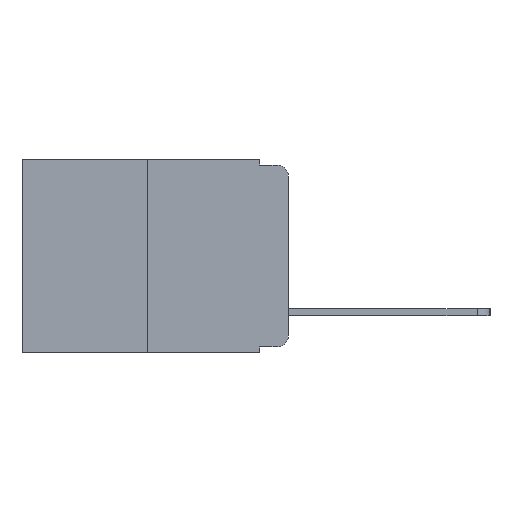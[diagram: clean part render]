
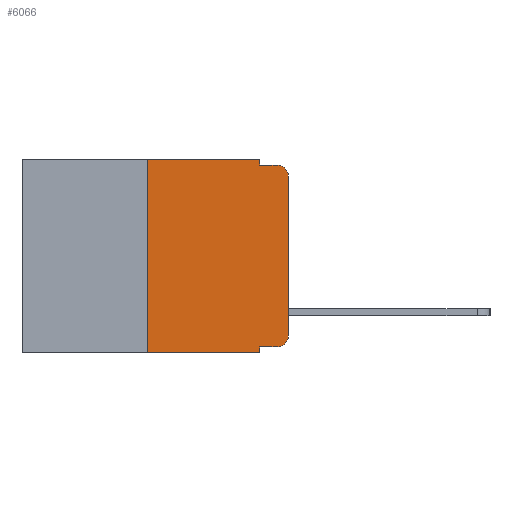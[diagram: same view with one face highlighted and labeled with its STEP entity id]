
A CAD part, left-side view. The second image highlights one B-rep face of the part: STEP entity #6066.
In plain terms, the highlighted planar face has unit normal (-1, 0, 0).
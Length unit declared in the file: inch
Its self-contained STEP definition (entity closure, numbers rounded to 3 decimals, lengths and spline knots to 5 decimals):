
#48 = DIRECTION ( 'NONE',  ( 0., 0., -1. ) ) ;
#591 = CARTESIAN_POINT ( 'NONE',  ( 0., 0.25, 0. ) ) ;
#1224 = FACE_OUTER_BOUND ( 'NONE', #18840, .T. ) ;
#1484 = DIRECTION ( 'NONE',  ( -1., 0., 0. ) ) ;
#1769 = CARTESIAN_POINT ( 'NONE',  ( 0., 0.051, -0.343 ) ) ;
#2409 = CARTESIAN_POINT ( 'NONE',  ( 0., 0.051, -0.01 ) ) ;
#2458 = EDGE_CURVE ( 'NONE', #11370, #16845, #17427, .T. ) ;
#2472 = ORIENTED_EDGE ( 'NONE', *, *, #4393, .F. ) ;
#2564 = CARTESIAN_POINT ( 'NONE',  ( 0., 0.051, -0.333 ) ) ;
#2819 = EDGE_CURVE ( 'NONE', #16101, #14282, #22959, .T. ) ;
#3037 = CARTESIAN_POINT ( 'NONE',  ( 0., 0.25, 0. ) ) ;
#3091 = CARTESIAN_POINT ( 'NONE',  ( 0., 0.02, -0.03 ) ) ;
#3475 = CIRCLE ( 'NONE', #16559, 0.02 ) ;
#3492 = CARTESIAN_POINT ( 'NONE',  ( 0., 0.02, -0.313 ) ) ;
#3577 = VECTOR ( 'NONE', #8615, 39.37008 ) ;
#3598 = ORIENTED_EDGE ( 'NONE', *, *, #7155, .F. ) ;
#4329 = ORIENTED_EDGE ( 'NONE', *, *, #2819, .F. ) ;
#4393 = EDGE_CURVE ( 'NONE', #19712, #17737, #8605, .T. ) ;
#4624 = CARTESIAN_POINT ( 'NONE',  ( 0., 0.02, -0.333 ) ) ;
#4773 = LINE ( 'NONE', #22912, #3577 ) ;
#4938 = DIRECTION ( 'NONE',  ( 0., 0., -1. ) ) ;
#5077 = ORIENTED_EDGE ( 'NONE', *, *, #21540, .T. ) ;
#5324 = EDGE_CURVE ( 'NONE', #16101, #6814, #19083, .T. ) ;
#5384 = CARTESIAN_POINT ( 'NONE',  ( 0., 0.02, -0.01 ) ) ;
#5534 = DIRECTION ( 'NONE',  ( 0., 0., -1. ) ) ;
#5817 = VECTOR ( 'NONE', #5534, 39.37008 ) ;
#6066 = ADVANCED_FACE ( 'NONE', ( #1224 ), #9665, .F. ) ;
#6263 = EDGE_CURVE ( 'NONE', #10305, #11370, #4773, .T. ) ;
#6814 = VERTEX_POINT ( 'NONE', #1769 ) ;
#7065 = ORIENTED_EDGE ( 'NONE', *, *, #15087, .F. ) ;
#7155 = EDGE_CURVE ( 'NONE', #8163, #19712, #21661, .T. ) ;
#7375 = VECTOR ( 'NONE', #8160, 39.37008 ) ;
#7403 = LINE ( 'NONE', #23131, #12507 ) ;
#8070 = VECTOR ( 'NONE', #18226, 39.37008 ) ;
#8160 = DIRECTION ( 'NONE',  ( 0., -1., 0. ) ) ;
#8163 = VERTEX_POINT ( 'NONE', #21022 ) ;
#8605 = LINE ( 'NONE', #2409, #7375 ) ;
#8615 = DIRECTION ( 'NONE',  ( 0., -1., 0. ) ) ;
#8666 = VECTOR ( 'NONE', #18124, 39.37008 ) ;
#9665 = PLANE ( 'NONE',  #14597 ) ;
#9990 = CARTESIAN_POINT ( 'NONE',  ( 0., 0., -0.313 ) ) ;
#10305 = VERTEX_POINT ( 'NONE', #2564 ) ;
#10750 = ORIENTED_EDGE ( 'NONE', *, *, #5324, .T. ) ;
#10871 = DIRECTION ( 'NONE',  ( 0., -1., 0. ) ) ;
#11062 = LINE ( 'NONE', #16855, #5817 ) ;
#11370 = VERTEX_POINT ( 'NONE', #4624 ) ;
#11606 = DIRECTION ( 'NONE',  ( 1., 0., 0. ) ) ;
#11610 = DIRECTION ( 'NONE',  ( 0., 0., -1. ) ) ;
#11843 = DIRECTION ( 'NONE',  ( 0., -1., 0. ) ) ;
#11847 = CARTESIAN_POINT ( 'NONE',  ( 0., 0.25, -0.343 ) ) ;
#12354 = VECTOR ( 'NONE', #23266, 39.37008 ) ;
#12507 = VECTOR ( 'NONE', #10871, 39.37008 ) ;
#12655 = AXIS2_PLACEMENT_3D ( 'NONE', #3492, #1484, #11610 ) ;
#13545 = CARTESIAN_POINT ( 'NONE',  ( 0., 0.051, -0.01 ) ) ;
#14282 = VERTEX_POINT ( 'NONE', #3037 ) ;
#14460 = VECTOR ( 'NONE', #11843, 39.37008 ) ;
#14597 = AXIS2_PLACEMENT_3D ( 'NONE', #22091, #11606, #48 ) ;
#14808 = ORIENTED_EDGE ( 'NONE', *, *, #15961, .F. ) ;
#15056 = EDGE_CURVE ( 'NONE', #16876, #17737, #3475, .T. ) ;
#15087 = EDGE_CURVE ( 'NONE', #14282, #8163, #7403, .T. ) ;
#15648 = CARTESIAN_POINT ( 'NONE',  ( 0., 0., -0.03 ) ) ;
#15794 = ORIENTED_EDGE ( 'NONE', *, *, #15056, .T. ) ;
#15961 = EDGE_CURVE ( 'NONE', #10305, #6814, #11062, .T. ) ;
#16101 = VERTEX_POINT ( 'NONE', #11847 ) ;
#16307 = DIRECTION ( 'NONE',  ( -1., 0., 0. ) ) ;
#16512 = CARTESIAN_POINT ( 'NONE',  ( 0., 0.051, 0. ) ) ;
#16559 = AXIS2_PLACEMENT_3D ( 'NONE', #3091, #16307, #4938 ) ;
#16845 = VERTEX_POINT ( 'NONE', #9990 ) ;
#16855 = CARTESIAN_POINT ( 'NONE',  ( 0., 0.051, 0. ) ) ;
#16876 = VERTEX_POINT ( 'NONE', #15648 ) ;
#17427 = CIRCLE ( 'NONE', #12655, 0.02 ) ;
#17737 = VERTEX_POINT ( 'NONE', #5384 ) ;
#18113 = ORIENTED_EDGE ( 'NONE', *, *, #6263, .T. ) ;
#18124 = DIRECTION ( 'NONE',  ( 0., 0., 1. ) ) ;
#18226 = DIRECTION ( 'NONE',  ( 0., 0., 1. ) ) ;
#18840 = EDGE_LOOP ( 'NONE', ( #5077, #15794, #2472, #3598, #7065, #4329, #10750, #14808, #18113, #23127 ) ) ;
#19083 = LINE ( 'NONE', #22314, #14460 ) ;
#19712 = VERTEX_POINT ( 'NONE', #13545 ) ;
#21022 = CARTESIAN_POINT ( 'NONE',  ( 0., 0.051, 0. ) ) ;
#21540 = EDGE_CURVE ( 'NONE', #16845, #16876, #21837, .T. ) ;
#21661 = LINE ( 'NONE', #16512, #12354 ) ;
#21837 = LINE ( 'NONE', #23133, #8666 ) ;
#22091 = CARTESIAN_POINT ( 'NONE',  ( 0., 0.473, 0. ) ) ;
#22314 = CARTESIAN_POINT ( 'NONE',  ( 0., 0.473, -0.343 ) ) ;
#22912 = CARTESIAN_POINT ( 'NONE',  ( 0., 0.051, -0.333 ) ) ;
#22959 = LINE ( 'NONE', #591, #8070 ) ;
#23127 = ORIENTED_EDGE ( 'NONE', *, *, #2458, .T. ) ;
#23131 = CARTESIAN_POINT ( 'NONE',  ( 0., 0.473, 0. ) ) ;
#23133 = CARTESIAN_POINT ( 'NONE',  ( 0., 0., 0. ) ) ;
#23266 = DIRECTION ( 'NONE',  ( 0., 0., -1. ) ) ;
